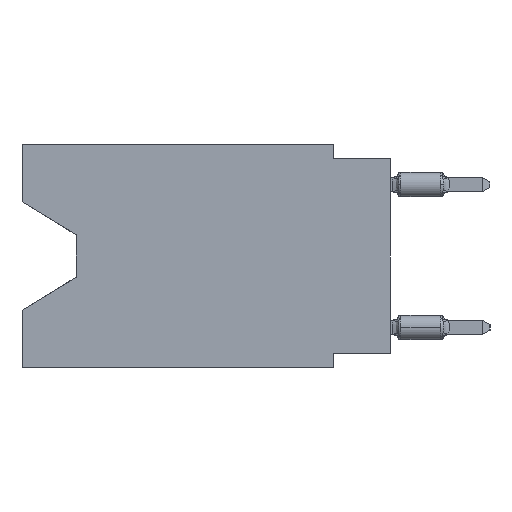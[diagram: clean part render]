
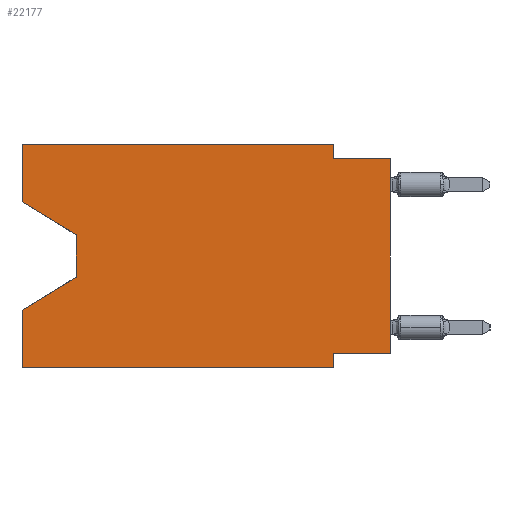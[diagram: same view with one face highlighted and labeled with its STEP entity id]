
A CAD part, left-side view. The second image highlights one B-rep face of the part: STEP entity #22177.
In plain terms, the highlighted planar face has unit normal (-1, 0, 0).
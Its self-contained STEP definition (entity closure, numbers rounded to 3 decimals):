
#528 = ORIENTED_EDGE ( 'NONE', *, *, #10040, .F. ) ;
#584 = ORIENTED_EDGE ( 'NONE', *, *, #39182, .T. ) ;
#633 = VECTOR ( 'NONE', #13298, 1000. ) ;
#842 = CARTESIAN_POINT ( 'NONE',  ( 0., 13.97, -5.893 ) ) ;
#1107 = CARTESIAN_POINT ( 'NONE',  ( 0., 2.54, -9.906 ) ) ;
#1251 = ORIENTED_EDGE ( 'NONE', *, *, #38135, .F. ) ;
#1544 = CARTESIAN_POINT ( 'NONE',  ( 0., 16.383, -2.546 ) ) ;
#2103 = FACE_OUTER_BOUND ( 'NONE', #34022, .T. ) ;
#2839 = LINE ( 'NONE', #26726, #5699 ) ;
#2977 = ORIENTED_EDGE ( 'NONE', *, *, #36932, .T. ) ;
#3031 = VERTEX_POINT ( 'NONE', #1107 ) ;
#3317 = VERTEX_POINT ( 'NONE', #30163 ) ;
#4448 = VERTEX_POINT ( 'NONE', #7286 ) ;
#5222 = CARTESIAN_POINT ( 'NONE',  ( 0., 13.97, -5.893 ) ) ;
#5312 = PLANE ( 'NONE',  #12515 ) ;
#5435 = CARTESIAN_POINT ( 'NONE',  ( 0., 2.54, -0.635 ) ) ;
#5562 = VECTOR ( 'NONE', #23425, 1000. ) ;
#5589 = LINE ( 'NONE', #23839, #5562 ) ;
#5699 = VECTOR ( 'NONE', #27305, 1000. ) ;
#5752 = CARTESIAN_POINT ( 'NONE',  ( 0., 16.383, 0. ) ) ;
#6034 = ORIENTED_EDGE ( 'NONE', *, *, #12958, .F. ) ;
#6099 = VERTEX_POINT ( 'NONE', #5435 ) ;
#6120 = CARTESIAN_POINT ( 'NONE',  ( 0., 13.97, -4.013 ) ) ;
#6727 = VECTOR ( 'NONE', #9502, 1000. ) ;
#7084 = ORIENTED_EDGE ( 'NONE', *, *, #36613, .F. ) ;
#7176 = ORIENTED_EDGE ( 'NONE', *, *, #10391, .F. ) ;
#7286 = CARTESIAN_POINT ( 'NONE',  ( 0., 16.383, -9.906 ) ) ;
#8713 = VECTOR ( 'NONE', #10049, 1000. ) ;
#9088 = EDGE_CURVE ( 'NONE', #23989, #11140, #10654, .T. ) ;
#9255 = VECTOR ( 'NONE', #26286, 1000. ) ;
#9311 = DIRECTION ( 'NONE',  ( 0., 0., 1. ) ) ;
#9502 = DIRECTION ( 'NONE',  ( 0., 0., 1. ) ) ;
#10040 = EDGE_CURVE ( 'NONE', #32028, #6099, #37040, .T. ) ;
#10049 = DIRECTION ( 'NONE',  ( 0., 1., 0. ) ) ;
#10391 = EDGE_CURVE ( 'NONE', #4448, #25043, #14966, .T. ) ;
#10584 = VERTEX_POINT ( 'NONE', #17473 ) ;
#10654 = LINE ( 'NONE', #38304, #9255 ) ;
#11140 = VERTEX_POINT ( 'NONE', #12225 ) ;
#11358 = DIRECTION ( 'NONE',  ( 1., 0., 0. ) ) ;
#12225 = CARTESIAN_POINT ( 'NONE',  ( 0., 16.383, 0. ) ) ;
#12515 = AXIS2_PLACEMENT_3D ( 'NONE', #38774, #11358, #23585 ) ;
#12958 = EDGE_CURVE ( 'NONE', #3317, #14084, #28072, .T. ) ;
#13298 = DIRECTION ( 'NONE',  ( 0., -1., 0. ) ) ;
#13422 = EDGE_CURVE ( 'NONE', #14084, #3031, #5589, .T. ) ;
#14084 = VERTEX_POINT ( 'NONE', #31965 ) ;
#14088 = CARTESIAN_POINT ( 'NONE',  ( 0., 16.383, -9.906 ) ) ;
#14456 = DIRECTION ( 'NONE',  ( 0., -1., 0. ) ) ;
#14484 = CARTESIAN_POINT ( 'NONE',  ( 0., 16.383, -7.36 ) ) ;
#14516 = VECTOR ( 'NONE', #33598, 1000. ) ;
#14966 = LINE ( 'NONE', #5752, #6727 ) ;
#15400 = LINE ( 'NONE', #21386, #14516 ) ;
#16393 = CARTESIAN_POINT ( 'NONE',  ( 0., 2.54, 0. ) ) ;
#16840 = EDGE_CURVE ( 'NONE', #29730, #30765, #33565, .T. ) ;
#17473 = CARTESIAN_POINT ( 'NONE',  ( 0., 0., -0.635 ) ) ;
#17608 = ORIENTED_EDGE ( 'NONE', *, *, #19494, .T. ) ;
#18158 = DIRECTION ( 'NONE',  ( 0., 0., -1. ) ) ;
#18345 = LINE ( 'NONE', #33963, #29755 ) ;
#19268 = CARTESIAN_POINT ( 'NONE',  ( 0., 0., -9.271 ) ) ;
#19494 = EDGE_CURVE ( 'NONE', #23989, #29730, #15400, .T. ) ;
#19781 = VECTOR ( 'NONE', #38893, 1000. ) ;
#21223 = ORIENTED_EDGE ( 'NONE', *, *, #9088, .F. ) ;
#21386 = CARTESIAN_POINT ( 'NONE',  ( 0., 16.383, -2.546 ) ) ;
#22177 = ADVANCED_FACE ( 'NONE', ( #2103 ), #5312, .F. ) ;
#22339 = VECTOR ( 'NONE', #18158, 1000. ) ;
#23425 = DIRECTION ( 'NONE',  ( 0., 0., -1. ) ) ;
#23473 = LINE ( 'NONE', #5222, #19781 ) ;
#23585 = DIRECTION ( 'NONE',  ( 0., 0., -1. ) ) ;
#23839 = CARTESIAN_POINT ( 'NONE',  ( 0., 2.54, -9.906 ) ) ;
#23989 = VERTEX_POINT ( 'NONE', #1544 ) ;
#25043 = VERTEX_POINT ( 'NONE', #14484 ) ;
#26091 = ORIENTED_EDGE ( 'NONE', *, *, #29022, .T. ) ;
#26286 = DIRECTION ( 'NONE',  ( 0., 0., 1. ) ) ;
#26726 = CARTESIAN_POINT ( 'NONE',  ( 0., 0., -0.635 ) ) ;
#27305 = DIRECTION ( 'NONE',  ( 0., -1., 0. ) ) ;
#28072 = LINE ( 'NONE', #19268, #8713 ) ;
#28659 = ORIENTED_EDGE ( 'NONE', *, *, #13422, .F. ) ;
#29022 = EDGE_CURVE ( 'NONE', #3317, #10584, #18345, .T. ) ;
#29279 = CARTESIAN_POINT ( 'NONE',  ( 0., 13.97, -4.013 ) ) ;
#29300 = LINE ( 'NONE', #14088, #633 ) ;
#29670 = CARTESIAN_POINT ( 'NONE',  ( 0., 16.383, 0. ) ) ;
#29730 = VERTEX_POINT ( 'NONE', #29279 ) ;
#29755 = VECTOR ( 'NONE', #9311, 1000. ) ;
#30163 = CARTESIAN_POINT ( 'NONE',  ( 0., 0., -9.271 ) ) ;
#30723 = VECTOR ( 'NONE', #14456, 1000. ) ;
#30765 = VERTEX_POINT ( 'NONE', #842 ) ;
#31886 = ORIENTED_EDGE ( 'NONE', *, *, #16840, .T. ) ;
#31965 = CARTESIAN_POINT ( 'NONE',  ( 0., 2.54, -9.271 ) ) ;
#32028 = VERTEX_POINT ( 'NONE', #37925 ) ;
#33565 = LINE ( 'NONE', #6120, #22339 ) ;
#33598 = DIRECTION ( 'NONE',  ( 0., -0.855, -0.519 ) ) ;
#33963 = CARTESIAN_POINT ( 'NONE',  ( 0., 0., 0. ) ) ;
#34022 = EDGE_LOOP ( 'NONE', ( #17608, #31886, #2977, #7176, #584, #28659, #6034, #26091, #7084, #528, #1251, #21223 ) ) ;
#34255 = VECTOR ( 'NONE', #34433, 1000. ) ;
#34433 = DIRECTION ( 'NONE',  ( 0., 0., -1. ) ) ;
#36613 = EDGE_CURVE ( 'NONE', #6099, #10584, #2839, .T. ) ;
#36932 = EDGE_CURVE ( 'NONE', #30765, #25043, #23473, .T. ) ;
#37040 = LINE ( 'NONE', #16393, #34255 ) ;
#37925 = CARTESIAN_POINT ( 'NONE',  ( 0., 2.54, 0. ) ) ;
#38135 = EDGE_CURVE ( 'NONE', #11140, #32028, #38901, .T. ) ;
#38304 = CARTESIAN_POINT ( 'NONE',  ( 0., 16.383, 0. ) ) ;
#38774 = CARTESIAN_POINT ( 'NONE',  ( 0., 16.383, 0. ) ) ;
#38893 = DIRECTION ( 'NONE',  ( 0., 0.855, -0.519 ) ) ;
#38901 = LINE ( 'NONE', #29670, #30723 ) ;
#39182 = EDGE_CURVE ( 'NONE', #4448, #3031, #29300, .T. ) ;
